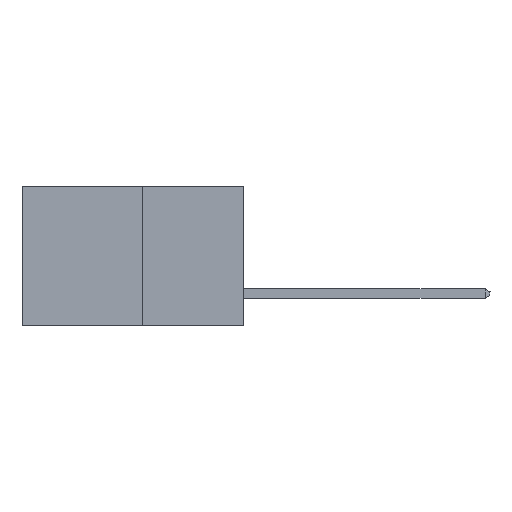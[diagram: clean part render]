
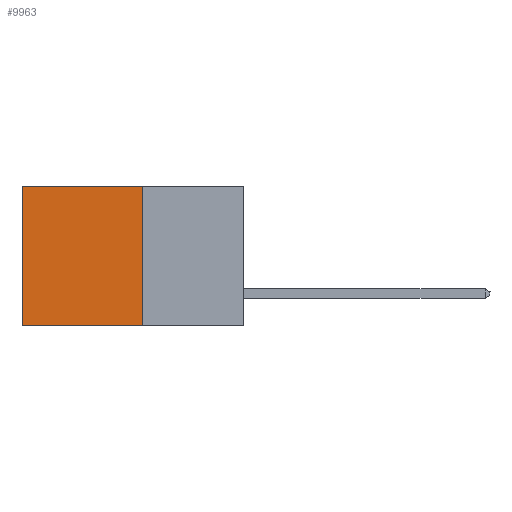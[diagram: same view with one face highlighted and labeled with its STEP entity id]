
A CAD part, left-side view. The second image highlights one B-rep face of the part: STEP entity #9963.
In plain terms, the highlighted planar face has unit normal (-1, 0, 0).
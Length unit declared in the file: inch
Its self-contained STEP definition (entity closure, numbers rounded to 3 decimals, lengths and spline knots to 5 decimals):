
#275 = EDGE_CURVE ( 'NONE', #11330, #10549, #11976, .T. ) ;
#361 = FACE_OUTER_BOUND ( 'NONE', #1563, .T. ) ;
#560 = CARTESIAN_POINT ( 'NONE',  ( 0.277, 0.59, 0. ) ) ;
#1174 = VECTOR ( 'NONE', #2718, 39.37008 ) ;
#1450 = CARTESIAN_POINT ( 'NONE',  ( 0.277, 0.27, 0. ) ) ;
#1563 = EDGE_LOOP ( 'NONE', ( #10066, #10670, #9204, #4943 ) ) ;
#1613 = PLANE ( 'NONE',  #7368 ) ;
#2718 = DIRECTION ( 'NONE',  ( 0., 1., 0. ) ) ;
#3090 = VERTEX_POINT ( 'NONE', #12732 ) ;
#4064 = CARTESIAN_POINT ( 'NONE',  ( 0.277, 0.27, 0. ) ) ;
#4094 = DIRECTION ( 'NONE',  ( 1., 0., 0. ) ) ;
#4943 = ORIENTED_EDGE ( 'NONE', *, *, #12017, .T. ) ;
#7140 = EDGE_CURVE ( 'NONE', #10549, #3090, #11239, .T. ) ;
#7295 = VERTEX_POINT ( 'NONE', #560 ) ;
#7368 = AXIS2_PLACEMENT_3D ( 'NONE', #11377, #4094, #12538 ) ;
#8410 = EDGE_CURVE ( 'NONE', #7295, #3090, #11018, .T. ) ;
#8792 = CARTESIAN_POINT ( 'NONE',  ( 0.277, 0.27, -0.37 ) ) ;
#9204 = ORIENTED_EDGE ( 'NONE', *, *, #275, .F. ) ;
#9963 = ADVANCED_FACE ( 'NONE', ( #361 ), #1613, .F. ) ;
#10066 = ORIENTED_EDGE ( 'NONE', *, *, #8410, .T. ) ;
#10088 = CARTESIAN_POINT ( 'NONE',  ( 0.277, 0.27, -0.37 ) ) ;
#10370 = CARTESIAN_POINT ( 'NONE',  ( 0.277, 0.59, -0.37 ) ) ;
#10549 = VERTEX_POINT ( 'NONE', #8792 ) ;
#10670 = ORIENTED_EDGE ( 'NONE', *, *, #7140, .F. ) ;
#11018 = LINE ( 'NONE', #10370, #13326 ) ;
#11239 = LINE ( 'NONE', #10088, #13550 ) ;
#11330 = VERTEX_POINT ( 'NONE', #4064 ) ;
#11377 = CARTESIAN_POINT ( 'NONE',  ( 0.277, 0.27, -0.37 ) ) ;
#11542 = DIRECTION ( 'NONE',  ( 0., 0., -1. ) ) ;
#11933 = DIRECTION ( 'NONE',  ( 0., 0., -1. ) ) ;
#11976 = LINE ( 'NONE', #12278, #14588 ) ;
#12017 = EDGE_CURVE ( 'NONE', #11330, #7295, #13599, .T. ) ;
#12278 = CARTESIAN_POINT ( 'NONE',  ( 0.277, 0.27, -0.37 ) ) ;
#12395 = DIRECTION ( 'NONE',  ( 0., 1., 0. ) ) ;
#12538 = DIRECTION ( 'NONE',  ( 0., 0., -1. ) ) ;
#12732 = CARTESIAN_POINT ( 'NONE',  ( 0.277, 0.59, -0.37 ) ) ;
#13326 = VECTOR ( 'NONE', #11542, 39.37008 ) ;
#13550 = VECTOR ( 'NONE', #12395, 39.37008 ) ;
#13599 = LINE ( 'NONE', #1450, #1174 ) ;
#14588 = VECTOR ( 'NONE', #11933, 39.37008 ) ;
